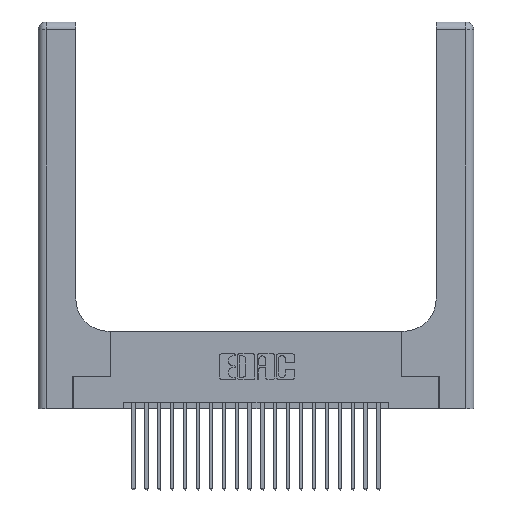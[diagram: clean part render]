
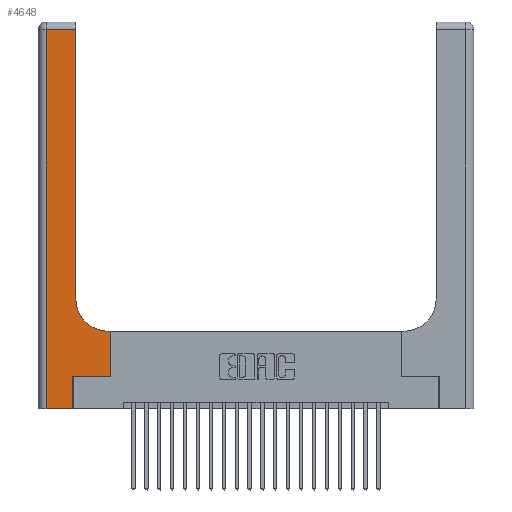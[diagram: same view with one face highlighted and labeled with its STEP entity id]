
A CAD part, top view. The second image highlights one B-rep face of the part: STEP entity #4648.
In plain terms, the highlighted planar face has unit normal (0, 0, 1).
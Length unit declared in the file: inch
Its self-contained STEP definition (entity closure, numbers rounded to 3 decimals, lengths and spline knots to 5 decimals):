
#358 = CARTESIAN_POINT ( 'NONE',  ( 0.269, 0., 0.37 ) ) ;
#829 = ORIENTED_EDGE ( 'NONE', *, *, #8610, .T. ) ;
#848 = EDGE_CURVE ( 'NONE', #10965, #6995, #18345, .T. ) ;
#890 = CARTESIAN_POINT ( 'NONE',  ( 0.06, 2.94, 0.37 ) ) ;
#1960 = CARTESIAN_POINT ( 'NONE',  ( 0.5585, 0.6, 0.37 ) ) ;
#2250 = DIRECTION ( 'NONE',  ( 0., 1., 0. ) ) ;
#3539 = ORIENTED_EDGE ( 'NONE', *, *, #13059, .T. ) ;
#3752 = ORIENTED_EDGE ( 'NONE', *, *, #848, .T. ) ;
#4216 = ORIENTED_EDGE ( 'NONE', *, *, #17658, .T. ) ;
#4648 = ADVANCED_FACE ( 'NONE', ( #8720 ), #8342, .F. ) ;
#4923 = DIRECTION ( 'NONE',  ( 1., 0., 0. ) ) ;
#5046 = CARTESIAN_POINT ( 'NONE',  ( 0., 0., 0.37 ) ) ;
#6292 = EDGE_CURVE ( 'NONE', #6995, #14495, #18077, .T. ) ;
#6511 = VECTOR ( 'NONE', #17806, 39.37008 ) ;
#6882 = DIRECTION ( 'NONE',  ( 1., 0., 0. ) ) ;
#6945 = VECTOR ( 'NONE', #4923, 39.37008 ) ;
#6995 = VERTEX_POINT ( 'NONE', #7984 ) ;
#7268 = ORIENTED_EDGE ( 'NONE', *, *, #6292, .T. ) ;
#7924 = LINE ( 'NONE', #19087, #21986 ) ;
#7984 = CARTESIAN_POINT ( 'NONE',  ( 0.5415, 0.6, 0.37 ) ) ;
#8038 = VECTOR ( 'NONE', #8511, 39.37008 ) ;
#8342 = PLANE ( 'NONE',  #12313 ) ;
#8396 = VERTEX_POINT ( 'NONE', #9161 ) ;
#8511 = DIRECTION ( 'NONE',  ( -1., 0., 0. ) ) ;
#8610 = EDGE_CURVE ( 'NONE', #23882, #8396, #23650, .T. ) ;
#8720 = FACE_OUTER_BOUND ( 'NONE', #20415, .T. ) ;
#8873 = CARTESIAN_POINT ( 'NONE',  ( 0.2915, 0.85, 0.37 ) ) ;
#8888 = EDGE_CURVE ( 'NONE', #8396, #16598, #17887, .T. ) ;
#9064 = VECTOR ( 'NONE', #6882, 39.37008 ) ;
#9161 = CARTESIAN_POINT ( 'NONE',  ( 0.269, 0.25, 0.37 ) ) ;
#9570 = CARTESIAN_POINT ( 'NONE',  ( 0.5415, 0.85, 0.37 ) ) ;
#10001 = VECTOR ( 'NONE', #21494, 39.37008 ) ;
#10200 = DIRECTION ( 'NONE',  ( 0., 0., -1. ) ) ;
#10536 = CARTESIAN_POINT ( 'NONE',  ( 0., 2.94, 0.37 ) ) ;
#10792 = LINE ( 'NONE', #5046, #9064 ) ;
#10965 = VERTEX_POINT ( 'NONE', #1960 ) ;
#11173 = LINE ( 'NONE', #13063, #11765 ) ;
#11396 = DIRECTION ( 'NONE',  ( 1., 0., 0. ) ) ;
#11765 = VECTOR ( 'NONE', #14929, 39.37008 ) ;
#12313 = AXIS2_PLACEMENT_3D ( 'NONE', #21148, #10200, #23022 ) ;
#12485 = AXIS2_PLACEMENT_3D ( 'NONE', #9570, #22379, #11396 ) ;
#12766 = VECTOR ( 'NONE', #2250, 39.37008 ) ;
#13059 = EDGE_CURVE ( 'NONE', #16598, #10965, #7924, .T. ) ;
#13063 = CARTESIAN_POINT ( 'NONE',  ( 0.06, 3., 0.37 ) ) ;
#13797 = CARTESIAN_POINT ( 'NONE',  ( 0.06, 0., 0.37 ) ) ;
#14131 = CARTESIAN_POINT ( 'NONE',  ( 0.269, 0.25, 0.37 ) ) ;
#14495 = VERTEX_POINT ( 'NONE', #8873 ) ;
#14929 = DIRECTION ( 'NONE',  ( 0., -1., 0. ) ) ;
#15079 = EDGE_CURVE ( 'NONE', #14495, #23346, #21188, .T. ) ;
#15162 = CARTESIAN_POINT ( 'NONE',  ( 0.269, 0., 0.37 ) ) ;
#16443 = EDGE_CURVE ( 'NONE', #23346, #22870, #19727, .T. ) ;
#16598 = VERTEX_POINT ( 'NONE', #18262 ) ;
#17526 = ORIENTED_EDGE ( 'NONE', *, *, #8888, .T. ) ;
#17658 = EDGE_CURVE ( 'NONE', #20579, #23882, #10792, .T. ) ;
#17673 = ORIENTED_EDGE ( 'NONE', *, *, #15079, .T. ) ;
#17806 = DIRECTION ( 'NONE',  ( 0., 1., 0. ) ) ;
#17887 = LINE ( 'NONE', #14131, #6945 ) ;
#18077 = CIRCLE ( 'NONE', #12485, 0.25 ) ;
#18262 = CARTESIAN_POINT ( 'NONE',  ( 0.5585, 0.25, 0.37 ) ) ;
#18285 = CARTESIAN_POINT ( 'NONE',  ( 0.2915, 0.6, 0.37 ) ) ;
#18345 = LINE ( 'NONE', #18285, #8038 ) ;
#19087 = CARTESIAN_POINT ( 'NONE',  ( 0.5585, 0.25, 0.37 ) ) ;
#19465 = ORIENTED_EDGE ( 'NONE', *, *, #23824, .T. ) ;
#19727 = LINE ( 'NONE', #10536, #10001 ) ;
#20415 = EDGE_LOOP ( 'NONE', ( #17673, #21067, #19465, #4216, #829, #17526, #3539, #3752, #7268 ) ) ;
#20579 = VERTEX_POINT ( 'NONE', #13797 ) ;
#21067 = ORIENTED_EDGE ( 'NONE', *, *, #16443, .T. ) ;
#21148 = CARTESIAN_POINT ( 'NONE',  ( 0., 3., 0.37 ) ) ;
#21188 = LINE ( 'NONE', #21329, #6511 ) ;
#21329 = CARTESIAN_POINT ( 'NONE',  ( 0.2915, 3., 0.37 ) ) ;
#21494 = DIRECTION ( 'NONE',  ( -1., 0., 0. ) ) ;
#21986 = VECTOR ( 'NONE', #22807, 39.37008 ) ;
#22379 = DIRECTION ( 'NONE',  ( 0., 0., -1. ) ) ;
#22796 = CARTESIAN_POINT ( 'NONE',  ( 0.2915, 2.94, 0.37 ) ) ;
#22807 = DIRECTION ( 'NONE',  ( 0., 1., 0. ) ) ;
#22870 = VERTEX_POINT ( 'NONE', #890 ) ;
#23022 = DIRECTION ( 'NONE',  ( -1., 0., 0. ) ) ;
#23346 = VERTEX_POINT ( 'NONE', #22796 ) ;
#23650 = LINE ( 'NONE', #358, #12766 ) ;
#23824 = EDGE_CURVE ( 'NONE', #22870, #20579, #11173, .T. ) ;
#23882 = VERTEX_POINT ( 'NONE', #15162 ) ;
